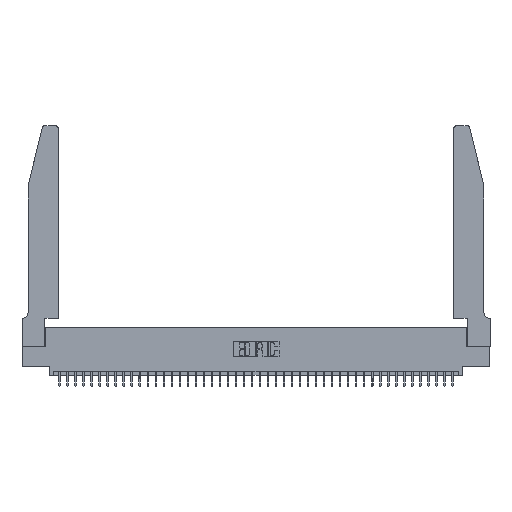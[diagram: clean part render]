
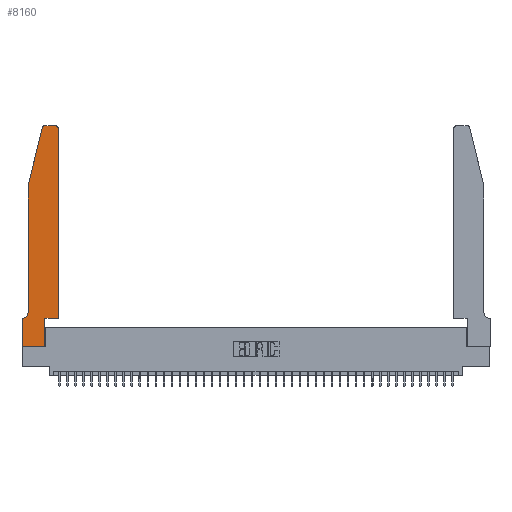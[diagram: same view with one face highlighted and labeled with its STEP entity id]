
A CAD part, top view. The second image highlights one B-rep face of the part: STEP entity #8160.
In plain terms, the highlighted planar face has unit normal (0, 0, 1).
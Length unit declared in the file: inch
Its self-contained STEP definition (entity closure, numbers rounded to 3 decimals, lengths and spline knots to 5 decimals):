
#134 = DIRECTION ( 'NONE',  ( 1., 0., 0. ) ) ;
#904 = VECTOR ( 'NONE', #31966, 39.37008 ) ;
#1016 = CARTESIAN_POINT ( 'NONE',  ( 0., 0., 0.37 ) ) ;
#1256 = CARTESIAN_POINT ( 'NONE',  ( 0.2865, 0.35, 0.37 ) ) ;
#1455 = EDGE_CURVE ( 'NONE', #32178, #30054, #6915, .T. ) ;
#1683 = CARTESIAN_POINT ( 'NONE',  ( 0.4505, 2.72, 0.37 ) ) ;
#1860 = VERTEX_POINT ( 'NONE', #13990 ) ;
#2408 = DIRECTION ( 'NONE',  ( 1., 0., 0. ) ) ;
#2410 = VECTOR ( 'NONE', #3782, 39.37008 ) ;
#2426 = CARTESIAN_POINT ( 'NONE',  ( 0.2865, 0.35, 0.37 ) ) ;
#2686 = EDGE_CURVE ( 'NONE', #9241, #31371, #9645, .T. ) ;
#2689 = ORIENTED_EDGE ( 'NONE', *, *, #1455, .T. ) ;
#2748 = LINE ( 'NONE', #13008, #25498 ) ;
#3782 = DIRECTION ( 'NONE',  ( -1., 0., 0. ) ) ;
#3874 = VERTEX_POINT ( 'NONE', #19871 ) ;
#3899 = DIRECTION ( 'NONE',  ( 0., 1., 0. ) ) ;
#3998 = CARTESIAN_POINT ( 'NONE',  ( 0.0755, 2., 0.37 ) ) ;
#4093 = CARTESIAN_POINT ( 'NONE',  ( 0.4505, 0.35, 0.37 ) ) ;
#4415 = ORIENTED_EDGE ( 'NONE', *, *, #25581, .T. ) ;
#5397 = PLANE ( 'NONE',  #19024 ) ;
#5968 = VECTOR ( 'NONE', #28220, 39.37008 ) ;
#6231 = CARTESIAN_POINT ( 'NONE',  ( 0.0755, 2., 0.37 ) ) ;
#6371 = CARTESIAN_POINT ( 'NONE',  ( 0.4205, 2.75, 0.37 ) ) ;
#6915 = CIRCLE ( 'NONE', #31348, 0.07 ) ;
#6935 = VECTOR ( 'NONE', #134, 39.37008 ) ;
#7021 = VERTEX_POINT ( 'NONE', #1016 ) ;
#7155 = AXIS2_PLACEMENT_3D ( 'NONE', #18997, #32358, #2408 ) ;
#8160 = ADVANCED_FACE ( 'NONE', ( #19134 ), #5397, .T. ) ;
#8490 = ORIENTED_EDGE ( 'NONE', *, *, #24397, .T. ) ;
#9112 = ORIENTED_EDGE ( 'NONE', *, *, #26428, .T. ) ;
#9241 = VERTEX_POINT ( 'NONE', #32053 ) ;
#9645 = CIRCLE ( 'NONE', #34082, 0.03 ) ;
#10570 = CARTESIAN_POINT ( 'NONE',  ( 0.0055, 0.42, 0.37 ) ) ;
#10784 = DIRECTION ( 'NONE',  ( -1., 0., 0. ) ) ;
#10907 = ORIENTED_EDGE ( 'NONE', *, *, #34914, .T. ) ;
#11085 = ORIENTED_EDGE ( 'NONE', *, *, #16749, .T. ) ;
#12805 = DIRECTION ( 'NONE',  ( 0., 0., 1. ) ) ;
#12879 = ORIENTED_EDGE ( 'NONE', *, *, #20189, .T. ) ;
#13008 = CARTESIAN_POINT ( 'NONE',  ( 0., 0., 0.37 ) ) ;
#13177 = EDGE_CURVE ( 'NONE', #3874, #32178, #27791, .T. ) ;
#13321 = CARTESIAN_POINT ( 'NONE',  ( 0.4505, 0.35, 0.37 ) ) ;
#13581 = CARTESIAN_POINT ( 'NONE',  ( 0.0755, 0.42, 0.37 ) ) ;
#13990 = CARTESIAN_POINT ( 'NONE',  ( 0.2865, 0., 0.37 ) ) ;
#14642 = ORIENTED_EDGE ( 'NONE', *, *, #13177, .T. ) ;
#14708 = VERTEX_POINT ( 'NONE', #6371 ) ;
#14812 = CIRCLE ( 'NONE', #7155, 0.03 ) ;
#15416 = CARTESIAN_POINT ( 'NONE',  ( 0., 0.35, 0.37 ) ) ;
#15652 = CARTESIAN_POINT ( 'NONE',  ( 0.284, 2.72, 0.37 ) ) ;
#16499 = ORIENTED_EDGE ( 'NONE', *, *, #40810, .T. ) ;
#16716 = LINE ( 'NONE', #30063, #6935 ) ;
#16749 = EDGE_CURVE ( 'NONE', #33078, #27688, #30333, .T. ) ;
#17135 = ORIENTED_EDGE ( 'NONE', *, *, #39268, .T. ) ;
#17315 = EDGE_CURVE ( 'NONE', #7021, #1860, #16716, .T. ) ;
#18997 = CARTESIAN_POINT ( 'NONE',  ( 0.4205, 2.72, 0.37 ) ) ;
#19024 = AXIS2_PLACEMENT_3D ( 'NONE', #15416, #12805, #26134 ) ;
#19134 = FACE_OUTER_BOUND ( 'NONE', #25116, .T. ) ;
#19871 = CARTESIAN_POINT ( 'NONE',  ( 0.0755, 2., 0.37 ) ) ;
#20189 = EDGE_CURVE ( 'NONE', #27688, #14708, #14812, .T. ) ;
#20652 = CARTESIAN_POINT ( 'NONE',  ( 0.0055, 0.35, 0.37 ) ) ;
#20790 = CARTESIAN_POINT ( 'NONE',  ( 0.0755, 0.35, 0.37 ) ) ;
#21863 = DIRECTION ( 'NONE',  ( 0., 1., 0. ) ) ;
#22143 = ORIENTED_EDGE ( 'NONE', *, *, #2686, .T. ) ;
#23865 = LINE ( 'NONE', #20790, #2410 ) ;
#24397 = EDGE_CURVE ( 'NONE', #30923, #33078, #40186, .T. ) ;
#25116 = EDGE_LOOP ( 'NONE', ( #17135, #22143, #10907, #14642, #2689, #16499, #9112, #41649, #4415, #8490, #11085, #12879 ) ) ;
#25498 = VECTOR ( 'NONE', #42490, 39.37008 ) ;
#25581 = EDGE_CURVE ( 'NONE', #1860, #30923, #32586, .T. ) ;
#25929 = DIRECTION ( 'NONE',  ( 1., 0., 0. ) ) ;
#26134 = DIRECTION ( 'NONE',  ( 1., 0., 0. ) ) ;
#26362 = CARTESIAN_POINT ( 'NONE',  ( 0., 0.35, 0.37 ) ) ;
#26428 = EDGE_CURVE ( 'NONE', #38667, #7021, #2748, .T. ) ;
#27688 = VERTEX_POINT ( 'NONE', #1683 ) ;
#27791 = LINE ( 'NONE', #3998, #5968 ) ;
#27819 = VECTOR ( 'NONE', #3899, 39.37008 ) ;
#28220 = DIRECTION ( 'NONE',  ( 0., -1., 0. ) ) ;
#28892 = CARTESIAN_POINT ( 'NONE',  ( 0.2605, 2.75, 0.37 ) ) ;
#29163 = DIRECTION ( 'NONE',  ( -0.239, -0.971, 0. ) ) ;
#29360 = DIRECTION ( 'NONE',  ( 0., 0., 1. ) ) ;
#29635 = VECTOR ( 'NONE', #21863, 39.37008 ) ;
#30054 = VERTEX_POINT ( 'NONE', #20652 ) ;
#30063 = CARTESIAN_POINT ( 'NONE',  ( 0., 0., 0.37 ) ) ;
#30333 = LINE ( 'NONE', #4093, #27819 ) ;
#30923 = VERTEX_POINT ( 'NONE', #1256 ) ;
#31348 = AXIS2_PLACEMENT_3D ( 'NONE', #10570, #40910, #10784 ) ;
#31371 = VERTEX_POINT ( 'NONE', #37501 ) ;
#31966 = DIRECTION ( 'NONE',  ( -1., 0., 0. ) ) ;
#32053 = CARTESIAN_POINT ( 'NONE',  ( 0.284, 2.75, 0.37 ) ) ;
#32178 = VERTEX_POINT ( 'NONE', #13581 ) ;
#32358 = DIRECTION ( 'NONE',  ( 0., 0., 1. ) ) ;
#32586 = LINE ( 'NONE', #2426, #29635 ) ;
#32900 = LINE ( 'NONE', #6231, #39729 ) ;
#33078 = VERTEX_POINT ( 'NONE', #38826 ) ;
#34082 = AXIS2_PLACEMENT_3D ( 'NONE', #15652, #29360, #25929 ) ;
#34914 = EDGE_CURVE ( 'NONE', #31371, #3874, #32900, .T. ) ;
#35882 = VECTOR ( 'NONE', #42815, 39.37008 ) ;
#37501 = CARTESIAN_POINT ( 'NONE',  ( 0.25487, 2.72718, 0.37 ) ) ;
#38507 = LINE ( 'NONE', #28892, #904 ) ;
#38667 = VERTEX_POINT ( 'NONE', #26362 ) ;
#38826 = CARTESIAN_POINT ( 'NONE',  ( 0.4505, 0.35, 0.37 ) ) ;
#39268 = EDGE_CURVE ( 'NONE', #14708, #9241, #38507, .T. ) ;
#39729 = VECTOR ( 'NONE', #29163, 39.37008 ) ;
#40186 = LINE ( 'NONE', #13321, #35882 ) ;
#40810 = EDGE_CURVE ( 'NONE', #30054, #38667, #23865, .T. ) ;
#40910 = DIRECTION ( 'NONE',  ( 0., 0., -1. ) ) ;
#41649 = ORIENTED_EDGE ( 'NONE', *, *, #17315, .T. ) ;
#42490 = DIRECTION ( 'NONE',  ( 0., -1., 0. ) ) ;
#42815 = DIRECTION ( 'NONE',  ( 1., 0., 0. ) ) ;
